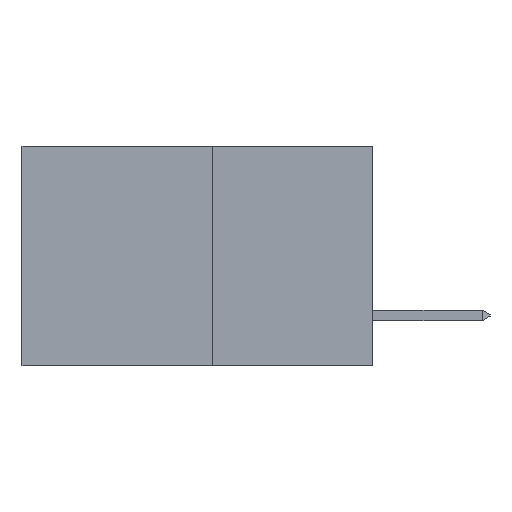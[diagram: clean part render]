
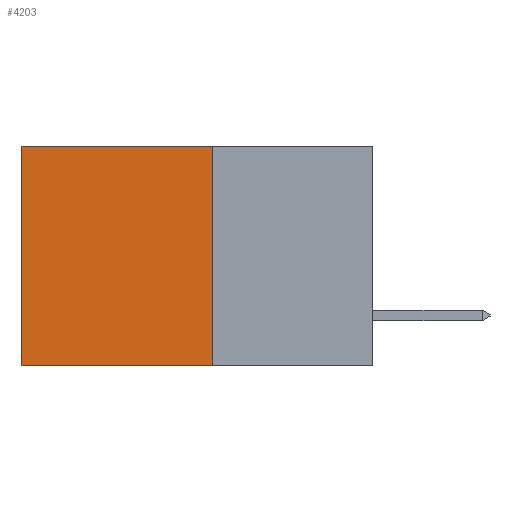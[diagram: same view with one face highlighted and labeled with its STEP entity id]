
A CAD part, left-side view. The second image highlights one B-rep face of the part: STEP entity #4203.
In plain terms, the highlighted planar face has unit normal (-1, 0, 0).
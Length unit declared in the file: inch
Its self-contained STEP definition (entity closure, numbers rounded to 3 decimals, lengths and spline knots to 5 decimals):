
#472 = VERTEX_POINT ( 'NONE', #14111 ) ;
#518 = FACE_OUTER_BOUND ( 'NONE', #14852, .T. ) ;
#756 = ORIENTED_EDGE ( 'NONE', *, *, #16405, .F. ) ;
#1225 = CARTESIAN_POINT ( 'NONE',  ( 0.277, 0.27, -0.37 ) ) ;
#1265 = VECTOR ( 'NONE', #21343, 39.37008 ) ;
#1290 = CARTESIAN_POINT ( 'NONE',  ( 0.277, 0.27, -0.37 ) ) ;
#1993 = LINE ( 'NONE', #1290, #10234 ) ;
#2937 = DIRECTION ( 'NONE',  ( 0., 1., 0. ) ) ;
#3527 = LINE ( 'NONE', #17448, #8416 ) ;
#3986 = LINE ( 'NONE', #6275, #12336 ) ;
#4203 = ADVANCED_FACE ( 'NONE', ( #518 ), #6767, .F. ) ;
#6223 = ORIENTED_EDGE ( 'NONE', *, *, #20882, .F. ) ;
#6275 = CARTESIAN_POINT ( 'NONE',  ( 0.277, 0.27, -0.37 ) ) ;
#6496 = AXIS2_PLACEMENT_3D ( 'NONE', #1225, #7040, #8398 ) ;
#6767 = PLANE ( 'NONE',  #6496 ) ;
#7040 = DIRECTION ( 'NONE',  ( 1., 0., 0. ) ) ;
#7792 = VERTEX_POINT ( 'NONE', #9840 ) ;
#8398 = DIRECTION ( 'NONE',  ( 0., 0., -1. ) ) ;
#8416 = VECTOR ( 'NONE', #20699, 39.37008 ) ;
#8782 = ORIENTED_EDGE ( 'NONE', *, *, #20265, .T. ) ;
#9840 = CARTESIAN_POINT ( 'NONE',  ( 0.277, 0.27, -0.37 ) ) ;
#10234 = VECTOR ( 'NONE', #2937, 39.37008 ) ;
#10392 = VERTEX_POINT ( 'NONE', #18696 ) ;
#10832 = VERTEX_POINT ( 'NONE', #13039 ) ;
#12336 = VECTOR ( 'NONE', #19699, 39.37008 ) ;
#13039 = CARTESIAN_POINT ( 'NONE',  ( 0.277, 0.27, 0. ) ) ;
#13979 = EDGE_CURVE ( 'NONE', #10832, #472, #3527, .T. ) ;
#14111 = CARTESIAN_POINT ( 'NONE',  ( 0.277, 0.59, 0. ) ) ;
#14852 = EDGE_LOOP ( 'NONE', ( #8782, #6223, #756, #16504 ) ) ;
#16405 = EDGE_CURVE ( 'NONE', #10832, #7792, #3986, .T. ) ;
#16502 = CARTESIAN_POINT ( 'NONE',  ( 0.277, 0.59, -0.37 ) ) ;
#16504 = ORIENTED_EDGE ( 'NONE', *, *, #13979, .T. ) ;
#17448 = CARTESIAN_POINT ( 'NONE',  ( 0.277, 0.27, 0. ) ) ;
#18696 = CARTESIAN_POINT ( 'NONE',  ( 0.277, 0.59, -0.37 ) ) ;
#19433 = LINE ( 'NONE', #16502, #1265 ) ;
#19699 = DIRECTION ( 'NONE',  ( 0., 0., -1. ) ) ;
#20265 = EDGE_CURVE ( 'NONE', #472, #10392, #19433, .T. ) ;
#20699 = DIRECTION ( 'NONE',  ( 0., 1., 0. ) ) ;
#20882 = EDGE_CURVE ( 'NONE', #7792, #10392, #1993, .T. ) ;
#21343 = DIRECTION ( 'NONE',  ( 0., 0., -1. ) ) ;
